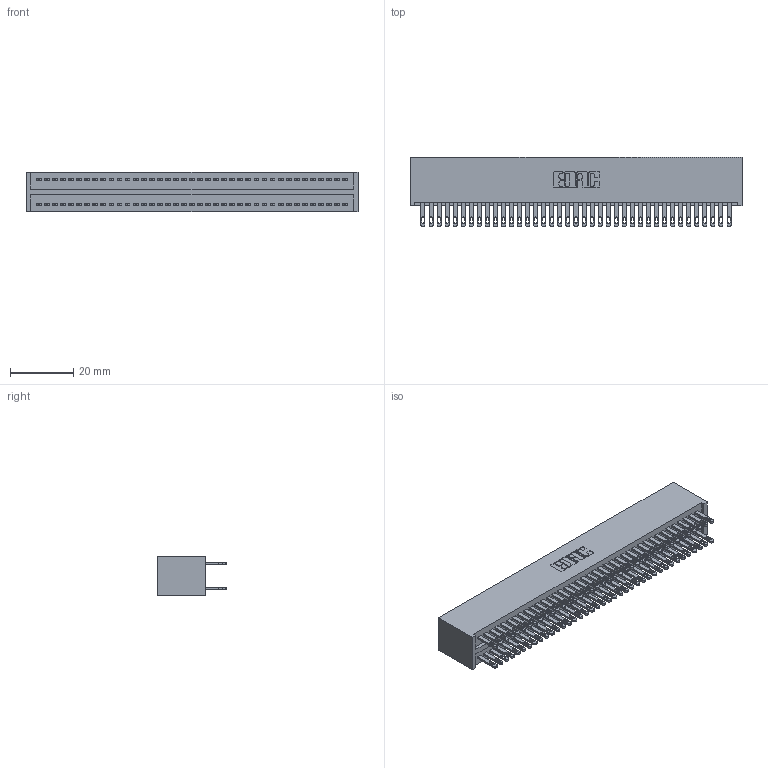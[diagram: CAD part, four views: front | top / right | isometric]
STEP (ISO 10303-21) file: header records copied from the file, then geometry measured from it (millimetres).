
FILE_DESCRIPTION (( 'STEP AP203' ), '1' );
FILE_NAME ('325-078-500-201.STEP', '2020-02-25T04:22:55', ( '' ), ( '' ), 'SwSTEP 2.0', 'SolidWorks 2016', '' );
FILE_SCHEMA (( 'CONFIG_CONTROL_DESIGN' ));
Length unit declared in the file: inch
Products named in the file (3): 325-292-001_325-293-100; 325-078-500-201; 325 Part_Lugless
Assembly tree (79 placements, depth 2):
  325-078-500-201
    325 Part_Lugless
    325-292-001_325-293-100  x78
Bounding box: 104.7 x 21.84 x 12.45 mm (x, y, z)
Volume: 14333.8 mm3; surface area: 18754.6 mm2
Topology: 79 solids, 79 shells, 3850 faces, 11753 edges, 7834 vertices
Faces by surface type: plane 2406, cylinder 1444
Entity records: 25131 total; most frequent: CARTESIAN_POINT 4166, ORIENTED_EDGE 4102, DIRECTION 3559, EDGE_CURVE 2051, LINE 1927, VECTOR 1927, VERTEX_POINT 1366, AXIS2_PLACEMENT_3D 816
